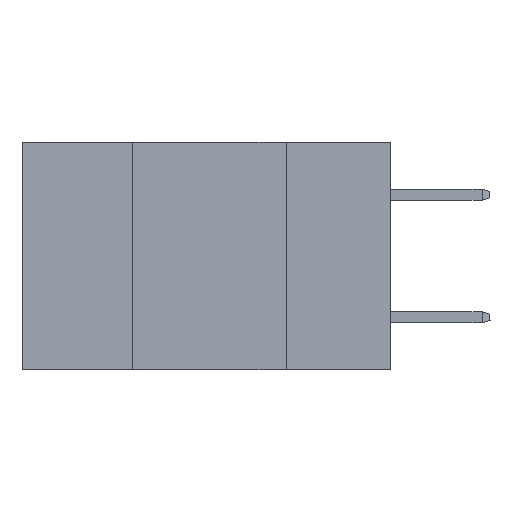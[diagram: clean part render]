
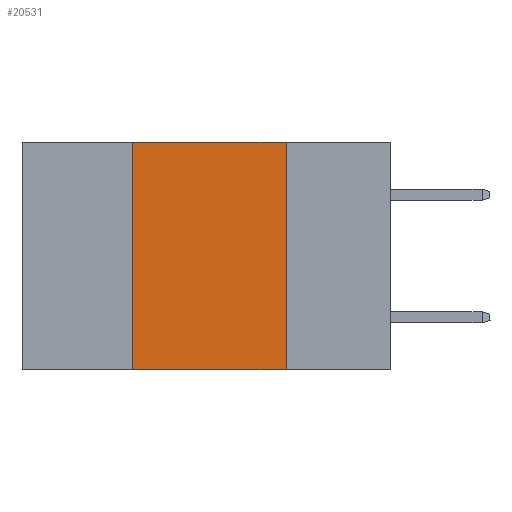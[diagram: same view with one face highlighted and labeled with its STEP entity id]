
A CAD part, left-side view. The second image highlights one B-rep face of the part: STEP entity #20531.
In plain terms, the highlighted planar face has unit normal (-1, 0, 0).
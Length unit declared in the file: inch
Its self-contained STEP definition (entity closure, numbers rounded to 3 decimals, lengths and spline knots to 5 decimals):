
#116 = LINE ( 'NONE', #13100, #16567 ) ;
#331 = LINE ( 'NONE', #2426, #21129 ) ;
#524 = PLANE ( 'NONE',  #31178 ) ;
#1960 = CARTESIAN_POINT ( 'NONE',  ( 0., 0.42, 0. ) ) ;
#2083 = ORIENTED_EDGE ( 'NONE', *, *, #28967, .T. ) ;
#2426 = CARTESIAN_POINT ( 'NONE',  ( 0., 0.6, 0. ) ) ;
#2763 = CARTESIAN_POINT ( 'NONE',  ( 0., 0.42, 0. ) ) ;
#3221 = DIRECTION ( 'NONE',  ( 0., 0., -1. ) ) ;
#5285 = CARTESIAN_POINT ( 'NONE',  ( 0., 0.42, -0.37 ) ) ;
#5746 = CARTESIAN_POINT ( 'NONE',  ( 0., 0.17, -0.37 ) ) ;
#5941 = VERTEX_POINT ( 'NONE', #5746 ) ;
#6009 = VECTOR ( 'NONE', #3221, 39.37008 ) ;
#6124 = VERTEX_POINT ( 'NONE', #2763 ) ;
#7966 = DIRECTION ( 'NONE',  ( 0., -1., 0. ) ) ;
#9336 = DIRECTION ( 'NONE',  ( 1., 0., 0. ) ) ;
#10488 = ORIENTED_EDGE ( 'NONE', *, *, #26802, .F. ) ;
#13003 = ORIENTED_EDGE ( 'NONE', *, *, #21602, .F. ) ;
#13100 = CARTESIAN_POINT ( 'NONE',  ( 0., 0.6, -0.37 ) ) ;
#15851 = VECTOR ( 'NONE', #30221, 39.37008 ) ;
#16047 = CARTESIAN_POINT ( 'NONE',  ( 0., 0.17, 0. ) ) ;
#16567 = VECTOR ( 'NONE', #21596, 39.37008 ) ;
#18812 = ORIENTED_EDGE ( 'NONE', *, *, #35474, .F. ) ;
#20531 = ADVANCED_FACE ( 'NONE', ( #32446 ), #524, .F. ) ;
#21129 = VECTOR ( 'NONE', #7966, 39.37008 ) ;
#21596 = DIRECTION ( 'NONE',  ( 0., -1., 0. ) ) ;
#21602 = EDGE_CURVE ( 'NONE', #30547, #5941, #25480, .T. ) ;
#23218 = CARTESIAN_POINT ( 'NONE',  ( 0., 0.17, 0. ) ) ;
#23244 = LINE ( 'NONE', #1960, #15851 ) ;
#25480 = LINE ( 'NONE', #16047, #6009 ) ;
#26802 = EDGE_CURVE ( 'NONE', #32959, #6124, #23244, .T. ) ;
#28720 = DIRECTION ( 'NONE',  ( 0., 0., -1. ) ) ;
#28967 = EDGE_CURVE ( 'NONE', #32959, #5941, #116, .T. ) ;
#30221 = DIRECTION ( 'NONE',  ( 0., 0., 1. ) ) ;
#30547 = VERTEX_POINT ( 'NONE', #23218 ) ;
#31097 = CARTESIAN_POINT ( 'NONE',  ( 0., 0.6, 0. ) ) ;
#31178 = AXIS2_PLACEMENT_3D ( 'NONE', #31097, #9336, #28720 ) ;
#32446 = FACE_OUTER_BOUND ( 'NONE', #35167, .T. ) ;
#32959 = VERTEX_POINT ( 'NONE', #5285 ) ;
#35167 = EDGE_LOOP ( 'NONE', ( #13003, #18812, #10488, #2083 ) ) ;
#35474 = EDGE_CURVE ( 'NONE', #6124, #30547, #331, .T. ) ;
